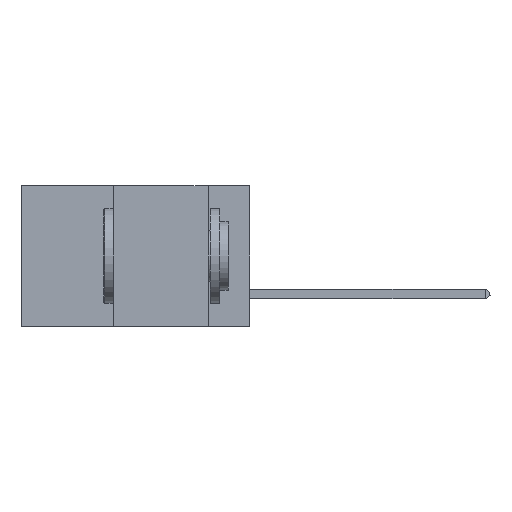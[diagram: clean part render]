
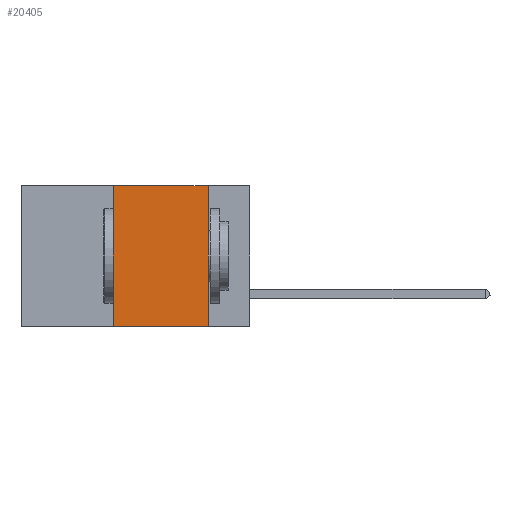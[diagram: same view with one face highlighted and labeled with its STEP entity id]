
A CAD part, left-side view. The second image highlights one B-rep face of the part: STEP entity #20405.
In plain terms, the highlighted planar face has unit normal (-1, 0, 0).
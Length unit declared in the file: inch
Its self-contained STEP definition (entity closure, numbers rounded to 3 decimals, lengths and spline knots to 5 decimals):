
#53 = DIRECTION ( 'NONE',  ( 0., 0., 1. ) ) ;
#430 = CARTESIAN_POINT ( 'NONE',  ( 0., 0.6, 0. ) ) ;
#816 = VERTEX_POINT ( 'NONE', #12966 ) ;
#939 = EDGE_LOOP ( 'NONE', ( #13197, #6366, #23693, #21638 ) ) ;
#1557 = AXIS2_PLACEMENT_3D ( 'NONE', #23117, #6820, #23043 ) ;
#1637 = VERTEX_POINT ( 'NONE', #21958 ) ;
#1724 = CARTESIAN_POINT ( 'NONE',  ( 0., 0.11, 0. ) ) ;
#1912 = CARTESIAN_POINT ( 'NONE',  ( 0., 0.6, -0.37 ) ) ;
#4329 = VECTOR ( 'NONE', #12848, 39.37008 ) ;
#4562 = VECTOR ( 'NONE', #20604, 39.37008 ) ;
#6366 = ORIENTED_EDGE ( 'NONE', *, *, #14376, .F. ) ;
#6491 = EDGE_CURVE ( 'NONE', #1637, #12429, #11489, .T. ) ;
#6820 = DIRECTION ( 'NONE',  ( 1., 0., 0. ) ) ;
#8101 = CARTESIAN_POINT ( 'NONE',  ( 0., 0.11, -0.37 ) ) ;
#8439 = CARTESIAN_POINT ( 'NONE',  ( 0., 0.36, 0. ) ) ;
#8713 = VECTOR ( 'NONE', #22080, 39.37008 ) ;
#9409 = LINE ( 'NONE', #430, #4562 ) ;
#10300 = LINE ( 'NONE', #1724, #4329 ) ;
#10879 = VECTOR ( 'NONE', #53, 39.37008 ) ;
#11489 = LINE ( 'NONE', #14886, #10879 ) ;
#12429 = VERTEX_POINT ( 'NONE', #8439 ) ;
#12848 = DIRECTION ( 'NONE',  ( 0., 0., -1. ) ) ;
#12966 = CARTESIAN_POINT ( 'NONE',  ( 0., 0.11, 0. ) ) ;
#13197 = ORIENTED_EDGE ( 'NONE', *, *, #18662, .F. ) ;
#14376 = EDGE_CURVE ( 'NONE', #12429, #816, #9409, .T. ) ;
#14476 = VERTEX_POINT ( 'NONE', #8101 ) ;
#14886 = CARTESIAN_POINT ( 'NONE',  ( 0., 0.36, 0. ) ) ;
#16778 = FACE_OUTER_BOUND ( 'NONE', #939, .T. ) ;
#17701 = PLANE ( 'NONE',  #1557 ) ;
#18662 = EDGE_CURVE ( 'NONE', #816, #14476, #10300, .T. ) ;
#20405 = ADVANCED_FACE ( 'NONE', ( #16778 ), #17701, .F. ) ;
#20604 = DIRECTION ( 'NONE',  ( 0., -1., 0. ) ) ;
#21344 = LINE ( 'NONE', #1912, #8713 ) ;
#21591 = EDGE_CURVE ( 'NONE', #1637, #14476, #21344, .T. ) ;
#21638 = ORIENTED_EDGE ( 'NONE', *, *, #21591, .T. ) ;
#21958 = CARTESIAN_POINT ( 'NONE',  ( 0., 0.36, -0.37 ) ) ;
#22080 = DIRECTION ( 'NONE',  ( 0., -1., 0. ) ) ;
#23043 = DIRECTION ( 'NONE',  ( 0., 0., -1. ) ) ;
#23117 = CARTESIAN_POINT ( 'NONE',  ( 0., 0.6, 0. ) ) ;
#23693 = ORIENTED_EDGE ( 'NONE', *, *, #6491, .F. ) ;
